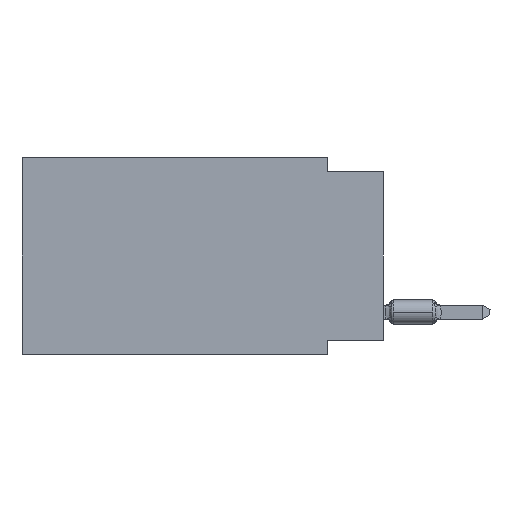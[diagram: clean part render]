
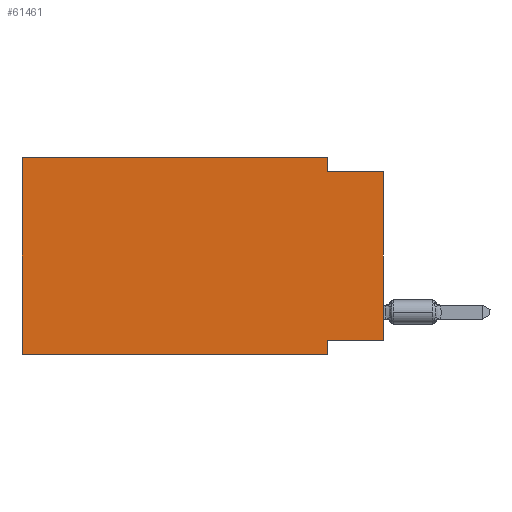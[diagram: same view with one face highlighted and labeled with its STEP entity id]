
A CAD part, left-side view. The second image highlights one B-rep face of the part: STEP entity #61461.
In plain terms, the highlighted planar face has unit normal (-1, 0, 0).
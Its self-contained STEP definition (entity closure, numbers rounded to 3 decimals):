
#321 = DIRECTION ( 'NONE',  ( 0., 0., -1. ) ) ;
#645 = CARTESIAN_POINT ( 'NONE',  ( 0., 0., -0.635 ) ) ;
#1725 = EDGE_CURVE ( 'NONE', #38927, #8149, #11128, .T. ) ;
#3222 = VERTEX_POINT ( 'NONE', #28303 ) ;
#3258 = DIRECTION ( 'NONE',  ( 0., -1., 0. ) ) ;
#3688 = ORIENTED_EDGE ( 'NONE', *, *, #25696, .F. ) ;
#4123 = PLANE ( 'NONE',  #39272 ) ;
#4650 = DIRECTION ( 'NONE',  ( 0., 0., -1. ) ) ;
#6913 = LINE ( 'NONE', #50869, #7091 ) ;
#7091 = VECTOR ( 'NONE', #41610, 1000. ) ;
#7165 = VECTOR ( 'NONE', #25157, 1000. ) ;
#8149 = VERTEX_POINT ( 'NONE', #645 ) ;
#8475 = DIRECTION ( 'NONE',  ( 0., -1., 0. ) ) ;
#10170 = CARTESIAN_POINT ( 'NONE',  ( 0., 0., -0.635 ) ) ;
#10813 = CARTESIAN_POINT ( 'NONE',  ( 0., 2.54, -8.89 ) ) ;
#10933 = EDGE_CURVE ( 'NONE', #59469, #45690, #12937, .T. ) ;
#11128 = LINE ( 'NONE', #49351, #7165 ) ;
#11942 = VECTOR ( 'NONE', #4650, 1000. ) ;
#12937 = LINE ( 'NONE', #61634, #13131 ) ;
#13131 = VECTOR ( 'NONE', #8475, 1000. ) ;
#14323 = DIRECTION ( 'NONE',  ( 0., 0., -1. ) ) ;
#16189 = EDGE_CURVE ( 'NONE', #47499, #59469, #41657, .T. ) ;
#18126 = LINE ( 'NONE', #33081, #33513 ) ;
#18134 = CARTESIAN_POINT ( 'NONE',  ( 0., 16.383, 0. ) ) ;
#18477 = VECTOR ( 'NONE', #321, 1000. ) ;
#20280 = ORIENTED_EDGE ( 'NONE', *, *, #30584, .F. ) ;
#20879 = ORIENTED_EDGE ( 'NONE', *, *, #21062, .F. ) ;
#21062 = EDGE_CURVE ( 'NONE', #41803, #8149, #34048, .T. ) ;
#22761 = VECTOR ( 'NONE', #55368, 1000. ) ;
#23374 = CARTESIAN_POINT ( 'NONE',  ( 0., 0., -8.255 ) ) ;
#23458 = CARTESIAN_POINT ( 'NONE',  ( 0., 2.54, 0. ) ) ;
#23775 = VERTEX_POINT ( 'NONE', #59847 ) ;
#25157 = DIRECTION ( 'NONE',  ( 0., 0., 1. ) ) ;
#25696 = EDGE_CURVE ( 'NONE', #45690, #41803, #43183, .T. ) ;
#28303 = CARTESIAN_POINT ( 'NONE',  ( 0., 2.54, -8.255 ) ) ;
#30584 = EDGE_CURVE ( 'NONE', #3222, #23775, #48104, .T. ) ;
#33081 = CARTESIAN_POINT ( 'NONE',  ( 0., 0., -8.255 ) ) ;
#33513 = VECTOR ( 'NONE', #57617, 1000. ) ;
#34048 = LINE ( 'NONE', #10170, #43392 ) ;
#34565 = ORIENTED_EDGE ( 'NONE', *, *, #58848, .T. ) ;
#38826 = DIRECTION ( 'NONE',  ( 1., 0., 0. ) ) ;
#38927 = VERTEX_POINT ( 'NONE', #23374 ) ;
#39272 = AXIS2_PLACEMENT_3D ( 'NONE', #18134, #38826, #14323 ) ;
#41014 = CARTESIAN_POINT ( 'NONE',  ( 0., 16.383, 0. ) ) ;
#41610 = DIRECTION ( 'NONE',  ( 0., -1., 0. ) ) ;
#41657 = LINE ( 'NONE', #41014, #22761 ) ;
#41803 = VERTEX_POINT ( 'NONE', #46495 ) ;
#43183 = LINE ( 'NONE', #23458, #11942 ) ;
#43392 = VECTOR ( 'NONE', #3258, 1000. ) ;
#44129 = ORIENTED_EDGE ( 'NONE', *, *, #16189, .F. ) ;
#45127 = ORIENTED_EDGE ( 'NONE', *, *, #58536, .F. ) ;
#45690 = VERTEX_POINT ( 'NONE', #59908 ) ;
#45703 = EDGE_LOOP ( 'NONE', ( #62316, #20879, #3688, #56661, #44129, #34565, #20280, #45127 ) ) ;
#46495 = CARTESIAN_POINT ( 'NONE',  ( 0., 2.54, -0.635 ) ) ;
#47499 = VERTEX_POINT ( 'NONE', #47731 ) ;
#47731 = CARTESIAN_POINT ( 'NONE',  ( 0., 16.383, -8.89 ) ) ;
#48104 = LINE ( 'NONE', #10813, #18477 ) ;
#49351 = CARTESIAN_POINT ( 'NONE',  ( 0., 0., 0. ) ) ;
#50869 = CARTESIAN_POINT ( 'NONE',  ( 0., 16.383, -8.89 ) ) ;
#55368 = DIRECTION ( 'NONE',  ( 0., 0., 1. ) ) ;
#56661 = ORIENTED_EDGE ( 'NONE', *, *, #10933, .F. ) ;
#57617 = DIRECTION ( 'NONE',  ( 0., 1., 0. ) ) ;
#58398 = CARTESIAN_POINT ( 'NONE',  ( 0., 16.383, 0. ) ) ;
#58536 = EDGE_CURVE ( 'NONE', #38927, #3222, #18126, .T. ) ;
#58848 = EDGE_CURVE ( 'NONE', #47499, #23775, #6913, .T. ) ;
#59469 = VERTEX_POINT ( 'NONE', #58398 ) ;
#59847 = CARTESIAN_POINT ( 'NONE',  ( 0., 2.54, -8.89 ) ) ;
#59908 = CARTESIAN_POINT ( 'NONE',  ( 0., 2.54, 0. ) ) ;
#61461 = ADVANCED_FACE ( 'NONE', ( #62393 ), #4123, .F. ) ;
#61634 = CARTESIAN_POINT ( 'NONE',  ( 0., 16.383, 0. ) ) ;
#62316 = ORIENTED_EDGE ( 'NONE', *, *, #1725, .T. ) ;
#62393 = FACE_OUTER_BOUND ( 'NONE', #45703, .T. ) ;
